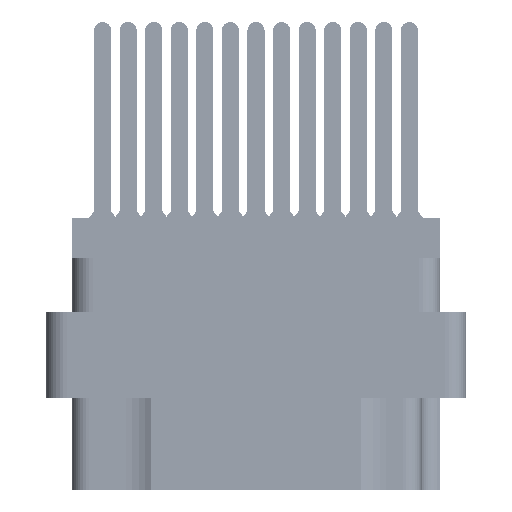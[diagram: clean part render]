
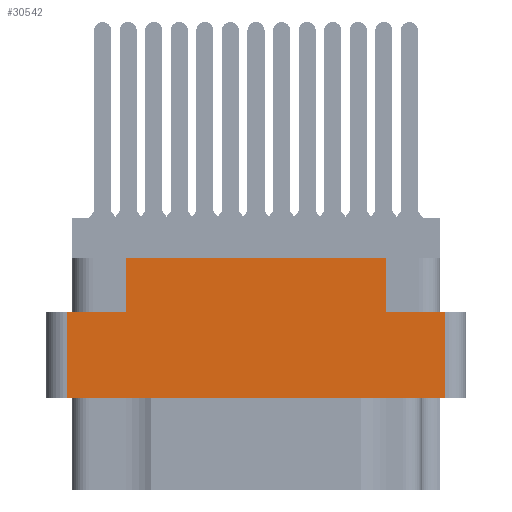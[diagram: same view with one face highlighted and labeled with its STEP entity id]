
A CAD part, left-side view. The second image highlights one B-rep face of the part: STEP entity #30542.
In plain terms, the highlighted planar face has unit normal (-1, 0, 0).
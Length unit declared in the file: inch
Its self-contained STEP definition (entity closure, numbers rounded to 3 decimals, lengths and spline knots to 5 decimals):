
#748 = LINE ( 'NONE', #37399, #49398 ) ;
#2093 = VECTOR ( 'NONE', #45300, 39.37008 ) ;
#2298 = LINE ( 'NONE', #47309, #45728 ) ;
#2368 = EDGE_CURVE ( 'NONE', #9405, #55099, #54992, .T. ) ;
#4685 = DIRECTION ( 'NONE',  ( 0., -1., 0. ) ) ;
#5006 = FACE_OUTER_BOUND ( 'NONE', #64325, .T. ) ;
#5148 = CARTESIAN_POINT ( 'NONE',  ( -1.359, -0.555, -0.277 ) ) ;
#5587 = CARTESIAN_POINT ( 'NONE',  ( -1.359, 0.3825, -0.117 ) ) ;
#5606 = EDGE_CURVE ( 'NONE', #64901, #55099, #748, .T. ) ;
#8108 = PLANE ( 'NONE',  #60283 ) ;
#8118 = CARTESIAN_POINT ( 'NONE',  ( -1.359, 0.555, -0.529 ) ) ;
#8913 = DIRECTION ( 'NONE',  ( 0., 1., 0. ) ) ;
#9052 = EDGE_CURVE ( 'NONE', #36416, #15319, #38664, .T. ) ;
#9405 = VERTEX_POINT ( 'NONE', #10311 ) ;
#9437 = ORIENTED_EDGE ( 'NONE', *, *, #38258, .F. ) ;
#10070 = EDGE_CURVE ( 'NONE', #9405, #66211, #57926, .T. ) ;
#10311 = CARTESIAN_POINT ( 'NONE',  ( -1.359, -0.3825, -0.277 ) ) ;
#11562 = VECTOR ( 'NONE', #47121, 39.37008 ) ;
#11973 = CARTESIAN_POINT ( 'NONE',  ( -1.359, -0.555, -0.529 ) ) ;
#12475 = DIRECTION ( 'NONE',  ( 0., 0., 1. ) ) ;
#15319 = VERTEX_POINT ( 'NONE', #5587 ) ;
#15425 = CARTESIAN_POINT ( 'NONE',  ( -1.359, 0.617, -0.117 ) ) ;
#16348 = DIRECTION ( 'NONE',  ( 0., 0., -1. ) ) ;
#16651 = ORIENTED_EDGE ( 'NONE', *, *, #22210, .F. ) ;
#21231 = DIRECTION ( 'NONE',  ( 0., 0., 1. ) ) ;
#22210 = EDGE_CURVE ( 'NONE', #15319, #66211, #65028, .T. ) ;
#22697 = DIRECTION ( 'NONE',  ( 0., 0., 1. ) ) ;
#23921 = CARTESIAN_POINT ( 'NONE',  ( -1.359, 0., -0.277 ) ) ;
#26121 = ORIENTED_EDGE ( 'NONE', *, *, #5606, .T. ) ;
#27099 = EDGE_CURVE ( 'NONE', #35247, #55925, #2298, .T. ) ;
#30542 = ADVANCED_FACE ( 'NONE', ( #5006 ), #8108, .T. ) ;
#33745 = ORIENTED_EDGE ( 'NONE', *, *, #70129, .F. ) ;
#35247 = VERTEX_POINT ( 'NONE', #60894 ) ;
#36416 = VERTEX_POINT ( 'NONE', #56070 ) ;
#37042 = CARTESIAN_POINT ( 'NONE',  ( -1.359, -0.3825, -0.117 ) ) ;
#37399 = CARTESIAN_POINT ( 'NONE',  ( -1.359, -0.555, -0.798 ) ) ;
#37465 = ORIENTED_EDGE ( 'NONE', *, *, #9052, .F. ) ;
#38258 = EDGE_CURVE ( 'NONE', #35247, #36416, #62548, .T. ) ;
#38664 = LINE ( 'NONE', #55793, #44624 ) ;
#40977 = DIRECTION ( 'NONE',  ( -1., 0., 0. ) ) ;
#41297 = CARTESIAN_POINT ( 'NONE',  ( -1.359, 0., -0.529 ) ) ;
#44624 = VECTOR ( 'NONE', #12475, 39.37008 ) ;
#45300 = DIRECTION ( 'NONE',  ( 0., -1., 0. ) ) ;
#45728 = VECTOR ( 'NONE', #16348, 39.37008 ) ;
#47121 = DIRECTION ( 'NONE',  ( 0., -1., 0. ) ) ;
#47309 = CARTESIAN_POINT ( 'NONE',  ( -1.359, 0.555, -0.798 ) ) ;
#47972 = VECTOR ( 'NONE', #4685, 39.37008 ) ;
#49398 = VECTOR ( 'NONE', #21231, 39.37008 ) ;
#49669 = ORIENTED_EDGE ( 'NONE', *, *, #27099, .T. ) ;
#54462 = VECTOR ( 'NONE', #8913, 39.37008 ) ;
#54852 = ORIENTED_EDGE ( 'NONE', *, *, #2368, .F. ) ;
#54992 = LINE ( 'NONE', #68545, #11562 ) ;
#55052 = CARTESIAN_POINT ( 'NONE',  ( -1.359, -0.3825, -0.277 ) ) ;
#55099 = VERTEX_POINT ( 'NONE', #5148 ) ;
#55793 = CARTESIAN_POINT ( 'NONE',  ( -1.359, 0.3825, -0.277 ) ) ;
#55925 = VERTEX_POINT ( 'NONE', #8118 ) ;
#56070 = CARTESIAN_POINT ( 'NONE',  ( -1.359, 0.3825, -0.277 ) ) ;
#57926 = LINE ( 'NONE', #55052, #64715 ) ;
#58572 = DIRECTION ( 'NONE',  ( 0., 0., 1. ) ) ;
#60283 = AXIS2_PLACEMENT_3D ( 'NONE', #68118, #40977, #58572 ) ;
#60894 = CARTESIAN_POINT ( 'NONE',  ( -1.359, 0.555, -0.277 ) ) ;
#62548 = LINE ( 'NONE', #23921, #2093 ) ;
#62984 = LINE ( 'NONE', #41297, #54462 ) ;
#64325 = EDGE_LOOP ( 'NONE', ( #9437, #49669, #33745, #26121, #54852, #67334, #16651, #37465 ) ) ;
#64715 = VECTOR ( 'NONE', #22697, 39.37008 ) ;
#64901 = VERTEX_POINT ( 'NONE', #11973 ) ;
#65028 = LINE ( 'NONE', #15425, #47972 ) ;
#66211 = VERTEX_POINT ( 'NONE', #37042 ) ;
#67334 = ORIENTED_EDGE ( 'NONE', *, *, #10070, .T. ) ;
#68118 = CARTESIAN_POINT ( 'NONE',  ( -1.359, -0.617, -0.798 ) ) ;
#68545 = CARTESIAN_POINT ( 'NONE',  ( -1.359, 0., -0.277 ) ) ;
#70129 = EDGE_CURVE ( 'NONE', #64901, #55925, #62984, .T. ) ;
